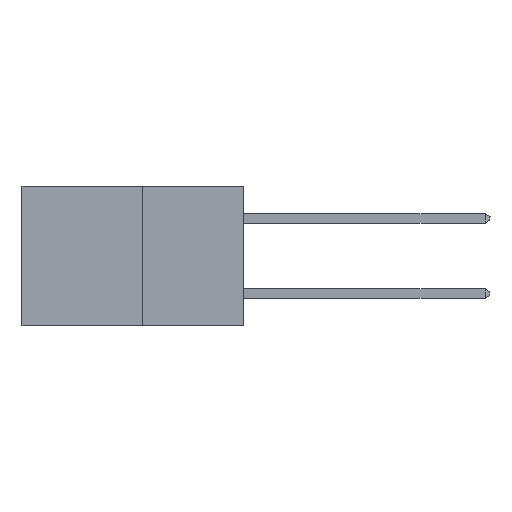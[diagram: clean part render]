
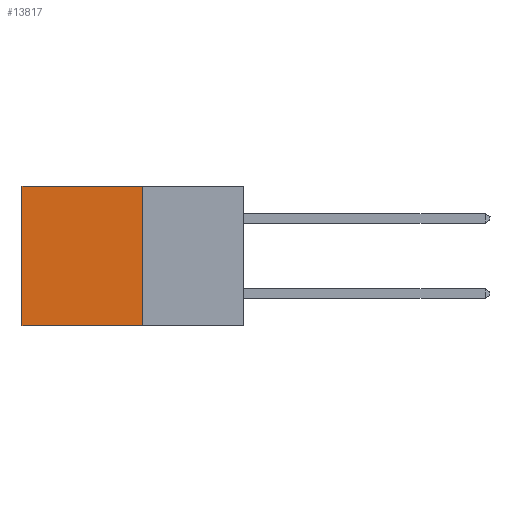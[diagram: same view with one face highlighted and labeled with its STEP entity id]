
A CAD part, left-side view. The second image highlights one B-rep face of the part: STEP entity #13817.
In plain terms, the highlighted planar face has unit normal (-1, 0, 0).
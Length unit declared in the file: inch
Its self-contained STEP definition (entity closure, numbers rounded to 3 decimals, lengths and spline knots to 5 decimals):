
#2 = ORIENTED_EDGE ( 'NONE', *, *, #6959, .T. ) ;
#87 = CARTESIAN_POINT ( 'NONE',  ( 0.277, 0.59, 0. ) ) ;
#232 = ORIENTED_EDGE ( 'NONE', *, *, #13619, .F. ) ;
#357 = LINE ( 'NONE', #2779, #7853 ) ;
#627 = DIRECTION ( 'NONE',  ( 0., 1., 0. ) ) ;
#714 = EDGE_CURVE ( 'NONE', #1710, #12524, #357, .T. ) ;
#926 = DIRECTION ( 'NONE',  ( 0., 1., 0. ) ) ;
#1004 = ORIENTED_EDGE ( 'NONE', *, *, #12087, .F. ) ;
#1186 = ORIENTED_EDGE ( 'NONE', *, *, #714, .T. ) ;
#1348 = DIRECTION ( 'NONE',  ( 1., 0., 0. ) ) ;
#1494 = LINE ( 'NONE', #13902, #1948 ) ;
#1710 = VERTEX_POINT ( 'NONE', #7635 ) ;
#1722 = FACE_OUTER_BOUND ( 'NONE', #3601, .T. ) ;
#1948 = VECTOR ( 'NONE', #926, 39.37008 ) ;
#2779 = CARTESIAN_POINT ( 'NONE',  ( 0.277, 0.27, 0. ) ) ;
#3341 = VECTOR ( 'NONE', #12074, 39.37008 ) ;
#3381 = VERTEX_POINT ( 'NONE', #9512 ) ;
#3601 = EDGE_LOOP ( 'NONE', ( #2, #232, #1004, #1186 ) ) ;
#5295 = LINE ( 'NONE', #6865, #14736 ) ;
#6807 = LINE ( 'NONE', #12071, #3341 ) ;
#6865 = CARTESIAN_POINT ( 'NONE',  ( 0.277, 0.27, -0.37 ) ) ;
#6959 = EDGE_CURVE ( 'NONE', #12524, #16365, #6807, .T. ) ;
#7635 = CARTESIAN_POINT ( 'NONE',  ( 0.277, 0.27, 0. ) ) ;
#7853 = VECTOR ( 'NONE', #627, 39.37008 ) ;
#8148 = DIRECTION ( 'NONE',  ( 0., 0., -1. ) ) ;
#9215 = CARTESIAN_POINT ( 'NONE',  ( 0.277, 0.27, -0.37 ) ) ;
#9512 = CARTESIAN_POINT ( 'NONE',  ( 0.277, 0.27, -0.37 ) ) ;
#10485 = DIRECTION ( 'NONE',  ( 0., 0., -1. ) ) ;
#11665 = PLANE ( 'NONE',  #15524 ) ;
#12071 = CARTESIAN_POINT ( 'NONE',  ( 0.277, 0.59, -0.37 ) ) ;
#12074 = DIRECTION ( 'NONE',  ( 0., 0., -1. ) ) ;
#12087 = EDGE_CURVE ( 'NONE', #1710, #3381, #5295, .T. ) ;
#12524 = VERTEX_POINT ( 'NONE', #87 ) ;
#13619 = EDGE_CURVE ( 'NONE', #3381, #16365, #1494, .T. ) ;
#13817 = ADVANCED_FACE ( 'NONE', ( #1722 ), #11665, .F. ) ;
#13902 = CARTESIAN_POINT ( 'NONE',  ( 0.277, 0.27, -0.37 ) ) ;
#14736 = VECTOR ( 'NONE', #8148, 39.37008 ) ;
#15524 = AXIS2_PLACEMENT_3D ( 'NONE', #9215, #1348, #10485 ) ;
#16135 = CARTESIAN_POINT ( 'NONE',  ( 0.277, 0.59, -0.37 ) ) ;
#16365 = VERTEX_POINT ( 'NONE', #16135 ) ;
